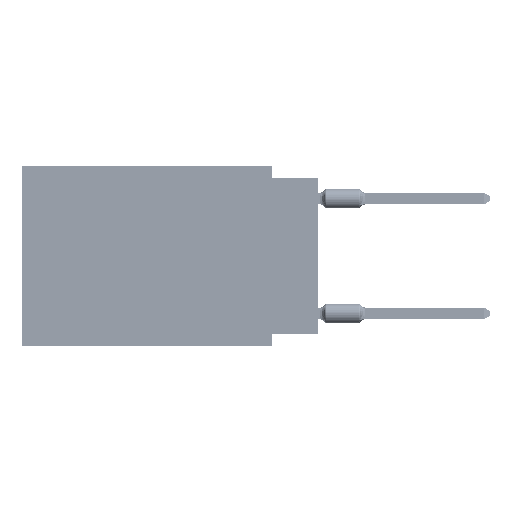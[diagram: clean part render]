
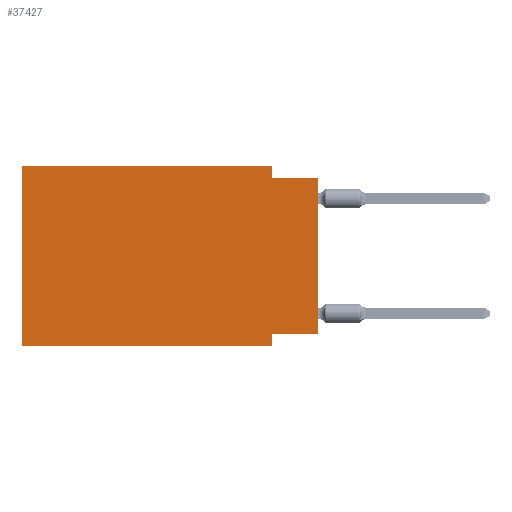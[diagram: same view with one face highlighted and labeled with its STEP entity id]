
A CAD part, left-side view. The second image highlights one B-rep face of the part: STEP entity #37427.
In plain terms, the highlighted planar face has unit normal (-1, 0, 0).
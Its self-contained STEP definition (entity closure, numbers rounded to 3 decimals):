
#652 = LINE ( 'NONE', #22340, #38278 ) ;
#1785 = CARTESIAN_POINT ( 'NONE',  ( 0., 0., -9.271 ) ) ;
#3167 = CARTESIAN_POINT ( 'NONE',  ( 0., 16.383, 0. ) ) ;
#4261 = CARTESIAN_POINT ( 'NONE',  ( 0., 2.54, -9.906 ) ) ;
#5045 = EDGE_CURVE ( 'NONE', #23690, #14794, #75256, .T. ) ;
#7251 = VECTOR ( 'NONE', #53297, 1000. ) ;
#8123 = DIRECTION ( 'NONE',  ( 0., 0., 1. ) ) ;
#9865 = FACE_OUTER_BOUND ( 'NONE', #13909, .T. ) ;
#9877 = LINE ( 'NONE', #33350, #7251 ) ;
#9990 = DIRECTION ( 'NONE',  ( 0., 0., 1. ) ) ;
#10015 = ORIENTED_EDGE ( 'NONE', *, *, #50721, .T. ) ;
#10745 = LINE ( 'NONE', #39974, #64412 ) ;
#10993 = CARTESIAN_POINT ( 'NONE',  ( 0., 16.383, 0. ) ) ;
#10994 = VECTOR ( 'NONE', #69941, 1000. ) ;
#11492 = LINE ( 'NONE', #23799, #10994 ) ;
#11710 = CARTESIAN_POINT ( 'NONE',  ( 0., 0., -0.635 ) ) ;
#13560 = VERTEX_POINT ( 'NONE', #3167 ) ;
#13909 = EDGE_LOOP ( 'NONE', ( #10015, #65361, #60343, #14691, #68466, #15338, #44752, #75861 ) ) ;
#14691 = ORIENTED_EDGE ( 'NONE', *, *, #46085, .F. ) ;
#14794 = VERTEX_POINT ( 'NONE', #56248 ) ;
#15338 = ORIENTED_EDGE ( 'NONE', *, *, #5045, .T. ) ;
#16033 = CARTESIAN_POINT ( 'NONE',  ( 0., 0., -0.635 ) ) ;
#17623 = CARTESIAN_POINT ( 'NONE',  ( 0., 2.54, -0.635 ) ) ;
#21397 = CARTESIAN_POINT ( 'NONE',  ( 0., 16.383, -9.906 ) ) ;
#22340 = CARTESIAN_POINT ( 'NONE',  ( 0., 2.54, 0. ) ) ;
#23690 = VERTEX_POINT ( 'NONE', #21397 ) ;
#23799 = CARTESIAN_POINT ( 'NONE',  ( 0., 0., -9.271 ) ) ;
#24136 = DIRECTION ( 'NONE',  ( 0., 0., -1. ) ) ;
#24835 = AXIS2_PLACEMENT_3D ( 'NONE', #10993, #51009, #69813 ) ;
#26053 = VECTOR ( 'NONE', #8123, 1000. ) ;
#28483 = EDGE_CURVE ( 'NONE', #23690, #13560, #65076, .T. ) ;
#28829 = EDGE_CURVE ( 'NONE', #68667, #57788, #652, .T. ) ;
#31786 = CARTESIAN_POINT ( 'NONE',  ( 0., 2.54, -9.271 ) ) ;
#32619 = VECTOR ( 'NONE', #70248, 1000. ) ;
#33350 = CARTESIAN_POINT ( 'NONE',  ( 0., 16.383, 0. ) ) ;
#33396 = VECTOR ( 'NONE', #34647, 1000. ) ;
#34647 = DIRECTION ( 'NONE',  ( 0., 0., -1. ) ) ;
#37427 = ADVANCED_FACE ( 'NONE', ( #9865 ), #69430, .F. ) ;
#38278 = VECTOR ( 'NONE', #24136, 1000. ) ;
#39521 = CARTESIAN_POINT ( 'NONE',  ( 0., 16.383, -9.906 ) ) ;
#39974 = CARTESIAN_POINT ( 'NONE',  ( 0., 0., 0. ) ) ;
#43988 = VECTOR ( 'NONE', #52480, 1000. ) ;
#44752 = ORIENTED_EDGE ( 'NONE', *, *, #73408, .F. ) ;
#46085 = EDGE_CURVE ( 'NONE', #13560, #68667, #9877, .T. ) ;
#48384 = EDGE_CURVE ( 'NONE', #70687, #63349, #11492, .T. ) ;
#50721 = EDGE_CURVE ( 'NONE', #70687, #58065, #10745, .T. ) ;
#51009 = DIRECTION ( 'NONE',  ( 1., 0., 0. ) ) ;
#52480 = DIRECTION ( 'NONE',  ( 0., -1., 0. ) ) ;
#53297 = DIRECTION ( 'NONE',  ( 0., -1., 0. ) ) ;
#53932 = CARTESIAN_POINT ( 'NONE',  ( 0., 16.383, 0. ) ) ;
#56248 = CARTESIAN_POINT ( 'NONE',  ( 0., 2.54, -9.906 ) ) ;
#56458 = LINE ( 'NONE', #11710, #43988 ) ;
#56957 = LINE ( 'NONE', #4261, #33396 ) ;
#57788 = VERTEX_POINT ( 'NONE', #17623 ) ;
#58065 = VERTEX_POINT ( 'NONE', #16033 ) ;
#60343 = ORIENTED_EDGE ( 'NONE', *, *, #28829, .F. ) ;
#63349 = VERTEX_POINT ( 'NONE', #31786 ) ;
#64412 = VECTOR ( 'NONE', #9990, 1000. ) ;
#65076 = LINE ( 'NONE', #53932, #26053 ) ;
#65361 = ORIENTED_EDGE ( 'NONE', *, *, #67973, .F. ) ;
#66547 = CARTESIAN_POINT ( 'NONE',  ( 0., 2.54, 0. ) ) ;
#67973 = EDGE_CURVE ( 'NONE', #57788, #58065, #56458, .T. ) ;
#68466 = ORIENTED_EDGE ( 'NONE', *, *, #28483, .F. ) ;
#68667 = VERTEX_POINT ( 'NONE', #66547 ) ;
#69430 = PLANE ( 'NONE',  #24835 ) ;
#69813 = DIRECTION ( 'NONE',  ( 0., 0., -1. ) ) ;
#69941 = DIRECTION ( 'NONE',  ( 0., 1., 0. ) ) ;
#70248 = DIRECTION ( 'NONE',  ( 0., -1., 0. ) ) ;
#70687 = VERTEX_POINT ( 'NONE', #1785 ) ;
#73408 = EDGE_CURVE ( 'NONE', #63349, #14794, #56957, .T. ) ;
#75256 = LINE ( 'NONE', #39521, #32619 ) ;
#75861 = ORIENTED_EDGE ( 'NONE', *, *, #48384, .F. ) ;
